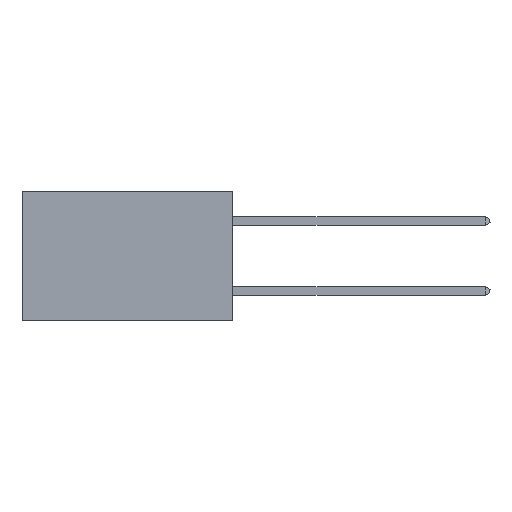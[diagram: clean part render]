
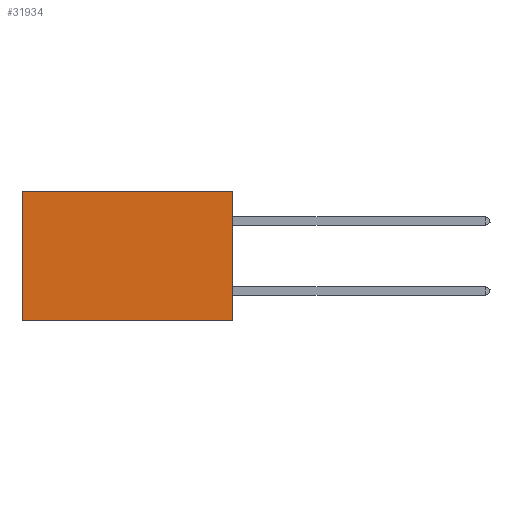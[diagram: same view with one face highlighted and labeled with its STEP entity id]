
A CAD part, left-side view. The second image highlights one B-rep face of the part: STEP entity #31934.
In plain terms, the highlighted planar face has unit normal (-1, 0, 0).
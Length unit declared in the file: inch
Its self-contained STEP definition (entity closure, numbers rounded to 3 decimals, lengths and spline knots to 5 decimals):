
#445 = VECTOR ( 'NONE', #25432, 39.37008 ) ;
#1794 = ORIENTED_EDGE ( 'NONE', *, *, #30288, .T. ) ;
#3464 = VECTOR ( 'NONE', #5945, 39.37008 ) ;
#5415 = CARTESIAN_POINT ( 'NONE',  ( 0.2875, 0., 0. ) ) ;
#5945 = DIRECTION ( 'NONE',  ( 0., 1., 0. ) ) ;
#7324 = EDGE_CURVE ( 'NONE', #10481, #15026, #11613, .T. ) ;
#9513 = AXIS2_PLACEMENT_3D ( 'NONE', #5415, #38704, #20829 ) ;
#9716 = ORIENTED_EDGE ( 'NONE', *, *, #33010, .F. ) ;
#10481 = VERTEX_POINT ( 'NONE', #35592 ) ;
#11545 = CARTESIAN_POINT ( 'NONE',  ( 0.2875, 0.6, -0.37 ) ) ;
#11598 = PLANE ( 'NONE',  #9513 ) ;
#11613 = LINE ( 'NONE', #18158, #3464 ) ;
#14081 = FACE_OUTER_BOUND ( 'NONE', #14493, .T. ) ;
#14493 = EDGE_LOOP ( 'NONE', ( #1794, #33360, #9716, #33315 ) ) ;
#15026 = VERTEX_POINT ( 'NONE', #28196 ) ;
#15147 = VERTEX_POINT ( 'NONE', #17301 ) ;
#16624 = VECTOR ( 'NONE', #37002, 39.37008 ) ;
#17301 = CARTESIAN_POINT ( 'NONE',  ( 0.2875, 0., -0.37 ) ) ;
#18158 = CARTESIAN_POINT ( 'NONE',  ( 0.2875, 0., 0. ) ) ;
#20829 = DIRECTION ( 'NONE',  ( 0., 0., -1. ) ) ;
#21363 = DIRECTION ( 'NONE',  ( 0., 0., -1. ) ) ;
#22436 = CARTESIAN_POINT ( 'NONE',  ( 0.2875, 0., -0.37 ) ) ;
#22538 = LINE ( 'NONE', #32823, #38431 ) ;
#25432 = DIRECTION ( 'NONE',  ( 0., 1., 0. ) ) ;
#27441 = EDGE_CURVE ( 'NONE', #15147, #34113, #32778, .T. ) ;
#28196 = CARTESIAN_POINT ( 'NONE',  ( 0.2875, 0.6, 0. ) ) ;
#30288 = EDGE_CURVE ( 'NONE', #15026, #34113, #32607, .T. ) ;
#31934 = ADVANCED_FACE ( 'NONE', ( #14081 ), #11598, .F. ) ;
#32607 = LINE ( 'NONE', #33986, #16624 ) ;
#32778 = LINE ( 'NONE', #22436, #445 ) ;
#32823 = CARTESIAN_POINT ( 'NONE',  ( 0.2875, 0., 0. ) ) ;
#33010 = EDGE_CURVE ( 'NONE', #10481, #15147, #22538, .T. ) ;
#33315 = ORIENTED_EDGE ( 'NONE', *, *, #7324, .T. ) ;
#33360 = ORIENTED_EDGE ( 'NONE', *, *, #27441, .F. ) ;
#33986 = CARTESIAN_POINT ( 'NONE',  ( 0.2875, 0.6, 0. ) ) ;
#34113 = VERTEX_POINT ( 'NONE', #11545 ) ;
#35592 = CARTESIAN_POINT ( 'NONE',  ( 0.2875, 0., 0. ) ) ;
#37002 = DIRECTION ( 'NONE',  ( 0., 0., -1. ) ) ;
#38431 = VECTOR ( 'NONE', #21363, 39.37008 ) ;
#38704 = DIRECTION ( 'NONE',  ( 1., 0., 0. ) ) ;
